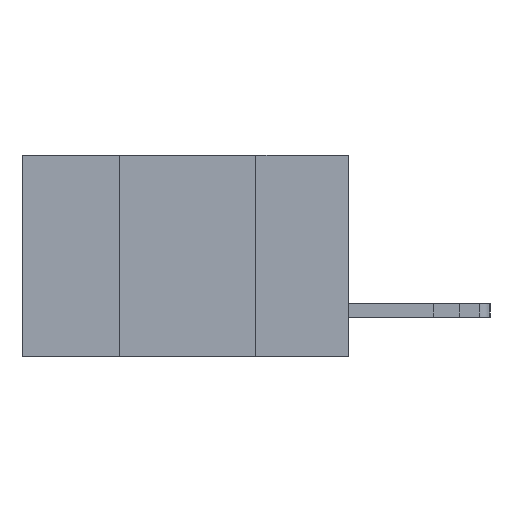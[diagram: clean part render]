
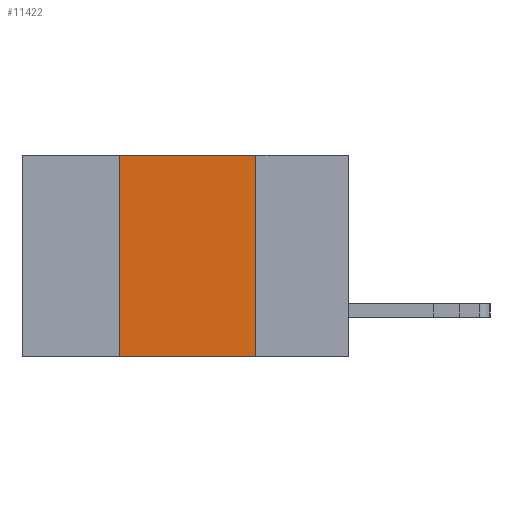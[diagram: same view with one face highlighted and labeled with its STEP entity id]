
A CAD part, left-side view. The second image highlights one B-rep face of the part: STEP entity #11422.
In plain terms, the highlighted planar face has unit normal (-1, 0, 0).
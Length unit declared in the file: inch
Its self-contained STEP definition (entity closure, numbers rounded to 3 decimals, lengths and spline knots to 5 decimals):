
#562 = CARTESIAN_POINT ( 'NONE',  ( 0., 0.17, 0. ) ) ;
#920 = LINE ( 'NONE', #22713, #10053 ) ;
#1188 = DIRECTION ( 'NONE',  ( 0., 0., 1. ) ) ;
#1204 = LINE ( 'NONE', #9114, #10314 ) ;
#1350 = DIRECTION ( 'NONE',  ( 0., 0., -1. ) ) ;
#1380 = DIRECTION ( 'NONE',  ( 1., 0., 0. ) ) ;
#1759 = VERTEX_POINT ( 'NONE', #22355 ) ;
#1961 = VERTEX_POINT ( 'NONE', #4232 ) ;
#3283 = DIRECTION ( 'NONE',  ( 0., 0., -1. ) ) ;
#3881 = CARTESIAN_POINT ( 'NONE',  ( 0., 0.6, 0. ) ) ;
#4232 = CARTESIAN_POINT ( 'NONE',  ( 0., 0.17, -0.37 ) ) ;
#4924 = ORIENTED_EDGE ( 'NONE', *, *, #5970, .F. ) ;
#5970 = EDGE_CURVE ( 'NONE', #8577, #9535, #1204, .T. ) ;
#8384 = LINE ( 'NONE', #15990, #12691 ) ;
#8577 = VERTEX_POINT ( 'NONE', #10769 ) ;
#9114 = CARTESIAN_POINT ( 'NONE',  ( 0., 0.6, 0. ) ) ;
#9161 = ORIENTED_EDGE ( 'NONE', *, *, #15336, .F. ) ;
#9356 = PLANE ( 'NONE',  #14679 ) ;
#9535 = VERTEX_POINT ( 'NONE', #562 ) ;
#9894 = VECTOR ( 'NONE', #17887, 39.37008 ) ;
#10053 = VECTOR ( 'NONE', #1188, 39.37008 ) ;
#10314 = VECTOR ( 'NONE', #17014, 39.37008 ) ;
#10769 = CARTESIAN_POINT ( 'NONE',  ( 0., 0.42, 0. ) ) ;
#10859 = ORIENTED_EDGE ( 'NONE', *, *, #18864, .T. ) ;
#11422 = ADVANCED_FACE ( 'NONE', ( #20520 ), #9356, .F. ) ;
#12691 = VECTOR ( 'NONE', #3283, 39.37008 ) ;
#14679 = AXIS2_PLACEMENT_3D ( 'NONE', #3881, #1380, #1350 ) ;
#15336 = EDGE_CURVE ( 'NONE', #1759, #8577, #920, .T. ) ;
#15959 = EDGE_LOOP ( 'NONE', ( #22275, #4924, #9161, #10859 ) ) ;
#15990 = CARTESIAN_POINT ( 'NONE',  ( 0., 0.17, 0. ) ) ;
#16044 = CARTESIAN_POINT ( 'NONE',  ( 0., 0.6, -0.37 ) ) ;
#17014 = DIRECTION ( 'NONE',  ( 0., -1., 0. ) ) ;
#17887 = DIRECTION ( 'NONE',  ( 0., -1., 0. ) ) ;
#18864 = EDGE_CURVE ( 'NONE', #1759, #1961, #19419, .T. ) ;
#19419 = LINE ( 'NONE', #16044, #9894 ) ;
#20520 = FACE_OUTER_BOUND ( 'NONE', #15959, .T. ) ;
#22275 = ORIENTED_EDGE ( 'NONE', *, *, #22368, .F. ) ;
#22355 = CARTESIAN_POINT ( 'NONE',  ( 0., 0.42, -0.37 ) ) ;
#22368 = EDGE_CURVE ( 'NONE', #9535, #1961, #8384, .T. ) ;
#22713 = CARTESIAN_POINT ( 'NONE',  ( 0., 0.42, 0. ) ) ;
